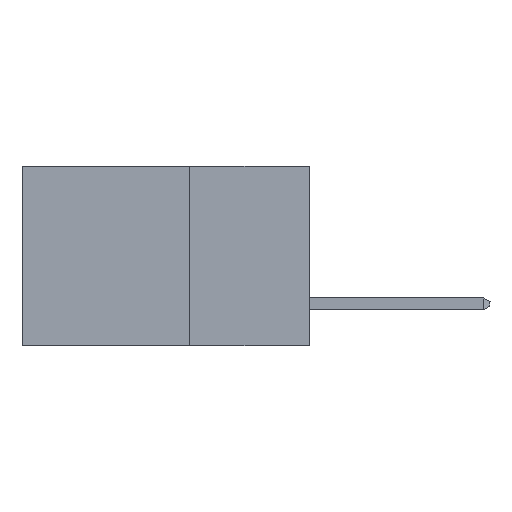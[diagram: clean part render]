
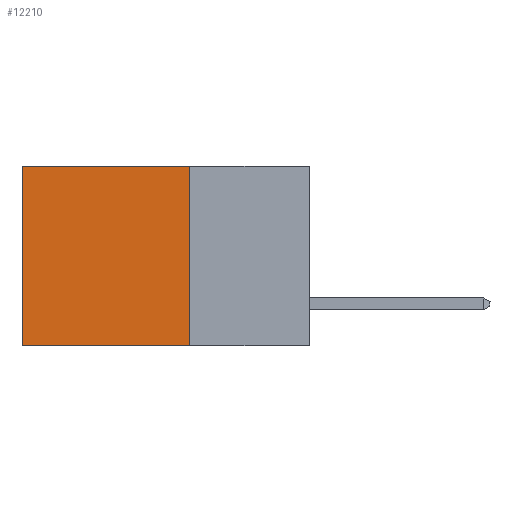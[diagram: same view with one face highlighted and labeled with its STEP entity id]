
A CAD part, left-side view. The second image highlights one B-rep face of the part: STEP entity #12210.
In plain terms, the highlighted planar face has unit normal (-1, 0, 0).
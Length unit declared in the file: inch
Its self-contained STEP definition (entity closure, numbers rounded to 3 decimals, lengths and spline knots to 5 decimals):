
#331 = DIRECTION ( 'NONE',  ( 0., 0., -1. ) ) ;
#583 = CARTESIAN_POINT ( 'NONE',  ( 0.2875, 0.6, -0.375 ) ) ;
#641 = ORIENTED_EDGE ( 'NONE', *, *, #5864, .T. ) ;
#1128 = VECTOR ( 'NONE', #3994, 39.37008 ) ;
#1470 = CARTESIAN_POINT ( 'NONE',  ( 0.2875, 0.25, 0. ) ) ;
#1479 = DIRECTION ( 'NONE',  ( 1., 0., 0. ) ) ;
#1826 = CARTESIAN_POINT ( 'NONE',  ( 0.2875, 0.25, -0.375 ) ) ;
#2830 = EDGE_LOOP ( 'NONE', ( #641, #9925, #7152, #13032 ) ) ;
#3232 = CARTESIAN_POINT ( 'NONE',  ( 0.2875, 0.6, 0. ) ) ;
#3994 = DIRECTION ( 'NONE',  ( 0., 0., -1. ) ) ;
#4043 = CARTESIAN_POINT ( 'NONE',  ( 0.2875, 0.6, -0.375 ) ) ;
#4490 = DIRECTION ( 'NONE',  ( 0., 1., 0. ) ) ;
#4501 = VERTEX_POINT ( 'NONE', #3232 ) ;
#5172 = CARTESIAN_POINT ( 'NONE',  ( 0.2875, 0.25, -0.375 ) ) ;
#5206 = VERTEX_POINT ( 'NONE', #14474 ) ;
#5530 = VECTOR ( 'NONE', #4490, 39.37008 ) ;
#5864 = EDGE_CURVE ( 'NONE', #4501, #13449, #11397, .T. ) ;
#6478 = CARTESIAN_POINT ( 'NONE',  ( 0.2875, 0.25, -0.375 ) ) ;
#6616 = AXIS2_PLACEMENT_3D ( 'NONE', #6478, #1479, #331 ) ;
#6795 = VECTOR ( 'NONE', #11641, 39.37008 ) ;
#7152 = ORIENTED_EDGE ( 'NONE', *, *, #9042, .F. ) ;
#7595 = LINE ( 'NONE', #1470, #6795 ) ;
#7651 = PLANE ( 'NONE',  #6616 ) ;
#9042 = EDGE_CURVE ( 'NONE', #5206, #16246, #13296, .T. ) ;
#9925 = ORIENTED_EDGE ( 'NONE', *, *, #11334, .F. ) ;
#9953 = VECTOR ( 'NONE', #10236, 39.37008 ) ;
#10236 = DIRECTION ( 'NONE',  ( 0., 0., -1. ) ) ;
#10633 = FACE_OUTER_BOUND ( 'NONE', #2830, .T. ) ;
#11334 = EDGE_CURVE ( 'NONE', #16246, #13449, #13592, .T. ) ;
#11397 = LINE ( 'NONE', #4043, #1128 ) ;
#11641 = DIRECTION ( 'NONE',  ( 0., 1., 0. ) ) ;
#12210 = ADVANCED_FACE ( 'NONE', ( #10633 ), #7651, .F. ) ;
#12658 = CARTESIAN_POINT ( 'NONE',  ( 0.2875, 0.25, -0.375 ) ) ;
#13032 = ORIENTED_EDGE ( 'NONE', *, *, #15475, .T. ) ;
#13296 = LINE ( 'NONE', #12658, #9953 ) ;
#13449 = VERTEX_POINT ( 'NONE', #583 ) ;
#13592 = LINE ( 'NONE', #1826, #5530 ) ;
#14474 = CARTESIAN_POINT ( 'NONE',  ( 0.2875, 0.25, 0. ) ) ;
#15475 = EDGE_CURVE ( 'NONE', #5206, #4501, #7595, .T. ) ;
#16246 = VERTEX_POINT ( 'NONE', #5172 ) ;
